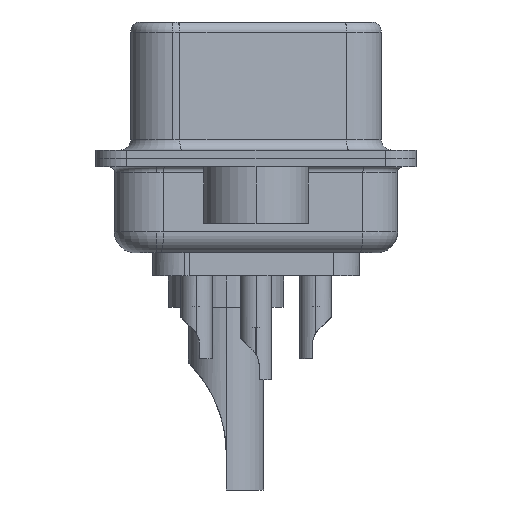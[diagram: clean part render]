
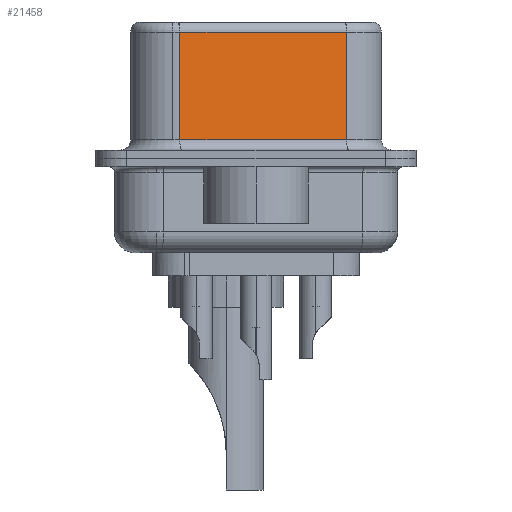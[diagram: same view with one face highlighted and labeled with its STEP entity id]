
A CAD part, left-side view. The second image highlights one B-rep face of the part: STEP entity #21458.
In plain terms, the highlighted planar face has unit normal (-0.985, -0.174, 0).
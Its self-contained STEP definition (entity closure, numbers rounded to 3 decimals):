
#797 = CARTESIAN_POINT ( 'NONE',  ( 5.132, -4.322, 6.52 ) ) ;
#981 = VERTEX_POINT ( 'NONE', #8035 ) ;
#990 = VECTOR ( 'NONE', #27984, 1000. ) ;
#1310 = LINE ( 'NONE', #6813, #13348 ) ;
#1665 = LINE ( 'NONE', #10712, #12976 ) ;
#3188 = DIRECTION ( 'NONE',  ( -0.174, 0.985, 0. ) ) ;
#4812 = DIRECTION ( 'NONE',  ( -0.174, 0.985, 0. ) ) ;
#4989 = ORIENTED_EDGE ( 'NONE', *, *, #13501, .F. ) ;
#5194 = AXIS2_PLACEMENT_3D ( 'NONE', #797, #16518, #3188 ) ;
#6089 = EDGE_CURVE ( 'NONE', #21805, #16987, #1310, .T. ) ;
#6813 = CARTESIAN_POINT ( 'NONE',  ( 5.132, -4.322, 6.02 ) ) ;
#7281 = VERTEX_POINT ( 'NONE', #9660 ) ;
#7715 = FACE_OUTER_BOUND ( 'NONE', #26350, .T. ) ;
#7944 = EDGE_CURVE ( 'NONE', #16987, #7281, #17649, .T. ) ;
#8035 = CARTESIAN_POINT ( 'NONE',  ( 5.132, -4.322, 0.9 ) ) ;
#9660 = CARTESIAN_POINT ( 'NONE',  ( 3.73, 3.628, 0.9 ) ) ;
#10712 = CARTESIAN_POINT ( 'NONE',  ( 5.132, -4.322, 6.52 ) ) ;
#12976 = VECTOR ( 'NONE', #21561, 1000. ) ;
#13348 = VECTOR ( 'NONE', #4812, 1000. ) ;
#13369 = CARTESIAN_POINT ( 'NONE',  ( 5.132, -4.322, 6.02 ) ) ;
#13501 = EDGE_CURVE ( 'NONE', #21805, #981, #1665, .T. ) ;
#14342 = PLANE ( 'NONE',  #5194 ) ;
#16518 = DIRECTION ( 'NONE',  ( 0.985, 0.174, 0. ) ) ;
#16978 = VECTOR ( 'NONE', #24937, 1000. ) ;
#16987 = VERTEX_POINT ( 'NONE', #25053 ) ;
#17649 = LINE ( 'NONE', #26196, #16978 ) ;
#18755 = LINE ( 'NONE', #23062, #990 ) ;
#20279 = ORIENTED_EDGE ( 'NONE', *, *, #6089, .T. ) ;
#20934 = ORIENTED_EDGE ( 'NONE', *, *, #28065, .T. ) ;
#21458 = ADVANCED_FACE ( 'NONE', ( #7715 ), #14342, .F. ) ;
#21561 = DIRECTION ( 'NONE',  ( 0., 0., -1. ) ) ;
#21805 = VERTEX_POINT ( 'NONE', #13369 ) ;
#23062 = CARTESIAN_POINT ( 'NONE',  ( 5.132, -4.322, 0.9 ) ) ;
#24937 = DIRECTION ( 'NONE',  ( 0., 0., -1. ) ) ;
#25053 = CARTESIAN_POINT ( 'NONE',  ( 3.73, 3.628, 6.02 ) ) ;
#26196 = CARTESIAN_POINT ( 'NONE',  ( 3.73, 3.628, 6.52 ) ) ;
#26350 = EDGE_LOOP ( 'NONE', ( #4989, #20279, #26846, #20934 ) ) ;
#26846 = ORIENTED_EDGE ( 'NONE', *, *, #7944, .T. ) ;
#27984 = DIRECTION ( 'NONE',  ( 0.174, -0.985, 0. ) ) ;
#28065 = EDGE_CURVE ( 'NONE', #7281, #981, #18755, .T. ) ;
